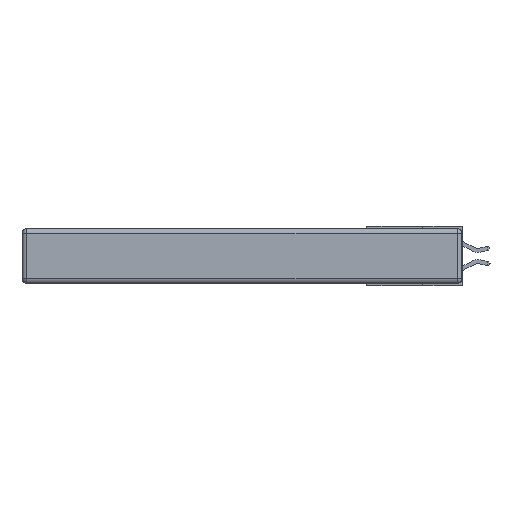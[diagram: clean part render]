
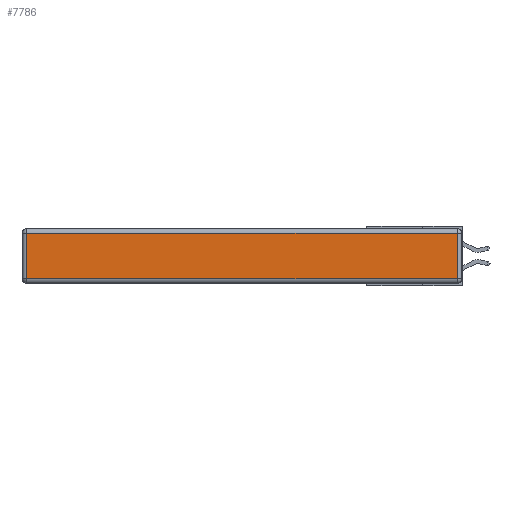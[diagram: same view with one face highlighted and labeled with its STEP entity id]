
A CAD part, left-side view. The second image highlights one B-rep face of the part: STEP entity #7786.
In plain terms, the highlighted planar face has unit normal (-1, 0, 0).
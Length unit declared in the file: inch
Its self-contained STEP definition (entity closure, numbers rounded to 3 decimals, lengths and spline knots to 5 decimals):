
#139 = LINE ( 'NONE', #1393, #9507 ) ;
#240 = DIRECTION ( 'NONE',  ( -1., 0., 0. ) ) ;
#797 = EDGE_CURVE ( 'NONE', #14223, #17735, #139, .T. ) ;
#1161 = CARTESIAN_POINT ( 'NONE',  ( 0., 2.72, -0.03 ) ) ;
#1393 = CARTESIAN_POINT ( 'NONE',  ( 0., 2.75, -0.03 ) ) ;
#2417 = ORIENTED_EDGE ( 'NONE', *, *, #8739, .T. ) ;
#2456 = VERTEX_POINT ( 'NONE', #9046 ) ;
#2568 = AXIS2_PLACEMENT_3D ( 'NONE', #8587, #240, #12818 ) ;
#3275 = ORIENTED_EDGE ( 'NONE', *, *, #797, .T. ) ;
#3583 = VECTOR ( 'NONE', #12863, 39.37008 ) ;
#4374 = PLANE ( 'NONE',  #2568 ) ;
#5654 = EDGE_LOOP ( 'NONE', ( #8580, #13101, #3275, #2417 ) ) ;
#7786 = ADVANCED_FACE ( 'NONE', ( #8540 ), #4374, .T. ) ;
#8068 = LINE ( 'NONE', #11294, #9148 ) ;
#8540 = FACE_OUTER_BOUND ( 'NONE', #5654, .T. ) ;
#8580 = ORIENTED_EDGE ( 'NONE', *, *, #12976, .T. ) ;
#8587 = CARTESIAN_POINT ( 'NONE',  ( 0., 0., -0.343 ) ) ;
#8628 = LINE ( 'NONE', #12311, #14080 ) ;
#8739 = EDGE_CURVE ( 'NONE', #17735, #11975, #15975, .T. ) ;
#9046 = CARTESIAN_POINT ( 'NONE',  ( 0., 0.03, -0.313 ) ) ;
#9148 = VECTOR ( 'NONE', #17142, 39.37008 ) ;
#9507 = VECTOR ( 'NONE', #12644, 39.37008 ) ;
#9621 = CARTESIAN_POINT ( 'NONE',  ( 0., 0.03, -0.03 ) ) ;
#10086 = CARTESIAN_POINT ( 'NONE',  ( 0., 2.72, -0.313 ) ) ;
#11294 = CARTESIAN_POINT ( 'NONE',  ( 0., 0.03, -0.343 ) ) ;
#11882 = EDGE_CURVE ( 'NONE', #2456, #14223, #8068, .T. ) ;
#11975 = VERTEX_POINT ( 'NONE', #10086 ) ;
#12311 = CARTESIAN_POINT ( 'NONE',  ( 0., 0., -0.313 ) ) ;
#12644 = DIRECTION ( 'NONE',  ( 0., 1., 0. ) ) ;
#12818 = DIRECTION ( 'NONE',  ( 0., 0., 1. ) ) ;
#12863 = DIRECTION ( 'NONE',  ( 0., 0., -1. ) ) ;
#12976 = EDGE_CURVE ( 'NONE', #11975, #2456, #8628, .T. ) ;
#13101 = ORIENTED_EDGE ( 'NONE', *, *, #11882, .T. ) ;
#14080 = VECTOR ( 'NONE', #16592, 39.37008 ) ;
#14223 = VERTEX_POINT ( 'NONE', #9621 ) ;
#15975 = LINE ( 'NONE', #17029, #3583 ) ;
#16592 = DIRECTION ( 'NONE',  ( 0., -1., 0. ) ) ;
#17029 = CARTESIAN_POINT ( 'NONE',  ( 0., 2.72, -0.343 ) ) ;
#17142 = DIRECTION ( 'NONE',  ( 0., 0., 1. ) ) ;
#17735 = VERTEX_POINT ( 'NONE', #1161 ) ;
